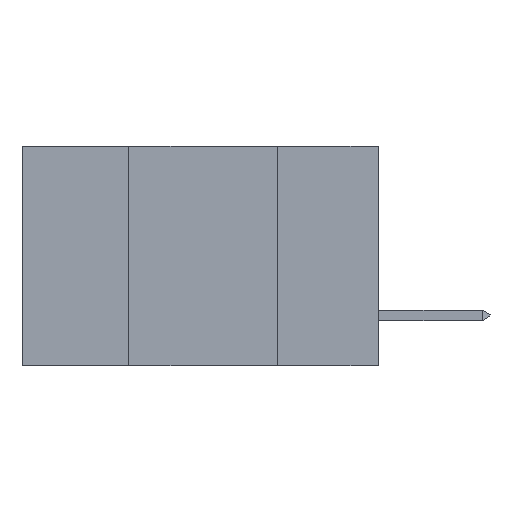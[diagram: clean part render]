
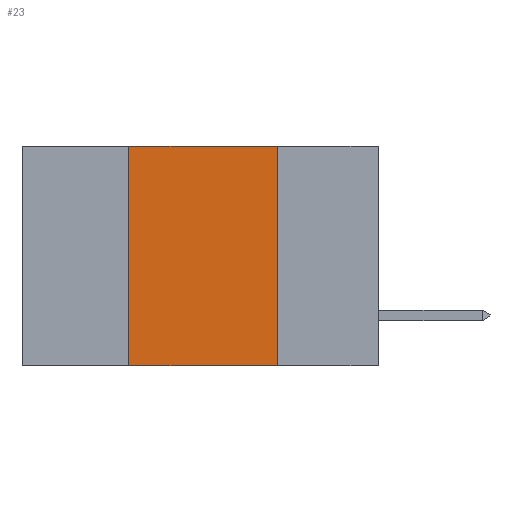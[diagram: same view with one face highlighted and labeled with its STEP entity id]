
A CAD part, left-side view. The second image highlights one B-rep face of the part: STEP entity #23.
In plain terms, the highlighted planar face has unit normal (-1, 0, 0).
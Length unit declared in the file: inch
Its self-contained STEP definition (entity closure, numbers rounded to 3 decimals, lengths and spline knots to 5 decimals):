
#23 = ADVANCED_FACE ( 'NONE', ( #6787 ), #5897, .F. ) ;
#663 = VECTOR ( 'NONE', #9480, 39.37008 ) ;
#1459 = EDGE_CURVE ( 'NONE', #3062, #4387, #8646, .T. ) ;
#1475 = EDGE_CURVE ( 'NONE', #5755, #4934, #2757, .T. ) ;
#1896 = VECTOR ( 'NONE', #6046, 39.37008 ) ;
#2667 = ORIENTED_EDGE ( 'NONE', *, *, #1459, .T. ) ;
#2757 = LINE ( 'NONE', #3622, #1896 ) ;
#3062 = VERTEX_POINT ( 'NONE', #3445 ) ;
#3445 = CARTESIAN_POINT ( 'NONE',  ( 0., 0.42, -0.37 ) ) ;
#3622 = CARTESIAN_POINT ( 'NONE',  ( 0., 0.6, 0. ) ) ;
#4142 = ORIENTED_EDGE ( 'NONE', *, *, #9244, .F. ) ;
#4161 = DIRECTION ( 'NONE',  ( 1., 0., 0. ) ) ;
#4241 = VECTOR ( 'NONE', #6585, 39.37008 ) ;
#4387 = VERTEX_POINT ( 'NONE', #8227 ) ;
#4934 = VERTEX_POINT ( 'NONE', #10618 ) ;
#5035 = CARTESIAN_POINT ( 'NONE',  ( 0., 0.6, 0. ) ) ;
#5254 = ORIENTED_EDGE ( 'NONE', *, *, #1475, .F. ) ;
#5261 = ORIENTED_EDGE ( 'NONE', *, *, #6847, .F. ) ;
#5755 = VERTEX_POINT ( 'NONE', #8969 ) ;
#5897 = PLANE ( 'NONE',  #6600 ) ;
#6046 = DIRECTION ( 'NONE',  ( 0., -1., 0. ) ) ;
#6585 = DIRECTION ( 'NONE',  ( 0., 0., -1. ) ) ;
#6600 = AXIS2_PLACEMENT_3D ( 'NONE', #5035, #4161, #8439 ) ;
#6730 = CARTESIAN_POINT ( 'NONE',  ( 0., 0.42, -0.37 ) ) ;
#6787 = FACE_OUTER_BOUND ( 'NONE', #7425, .T. ) ;
#6847 = EDGE_CURVE ( 'NONE', #3062, #5755, #9057, .T. ) ;
#7425 = EDGE_LOOP ( 'NONE', ( #4142, #5254, #5261, #2667 ) ) ;
#7973 = VECTOR ( 'NONE', #9216, 39.37008 ) ;
#8227 = CARTESIAN_POINT ( 'NONE',  ( 0., 0.17, -0.37 ) ) ;
#8439 = DIRECTION ( 'NONE',  ( 0., 0., -1. ) ) ;
#8646 = LINE ( 'NONE', #9640, #663 ) ;
#8853 = CARTESIAN_POINT ( 'NONE',  ( 0., 0.17, -0.37 ) ) ;
#8969 = CARTESIAN_POINT ( 'NONE',  ( 0., 0.42, 0. ) ) ;
#9057 = LINE ( 'NONE', #6730, #7973 ) ;
#9216 = DIRECTION ( 'NONE',  ( 0., 0., 1. ) ) ;
#9244 = EDGE_CURVE ( 'NONE', #4934, #4387, #10512, .T. ) ;
#9480 = DIRECTION ( 'NONE',  ( 0., -1., 0. ) ) ;
#9640 = CARTESIAN_POINT ( 'NONE',  ( 0., 0.6, -0.37 ) ) ;
#10512 = LINE ( 'NONE', #8853, #4241 ) ;
#10618 = CARTESIAN_POINT ( 'NONE',  ( 0., 0.17, 0. ) ) ;
